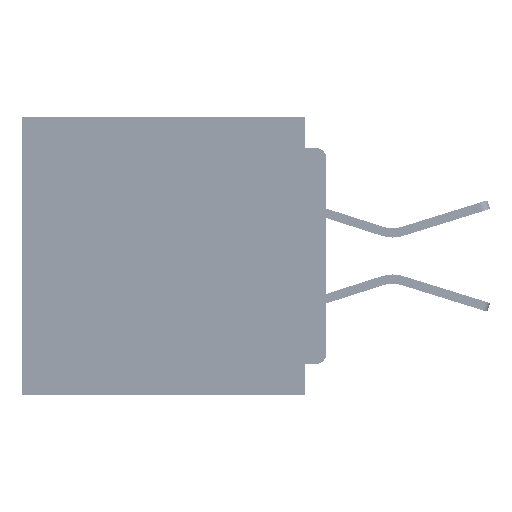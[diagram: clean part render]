
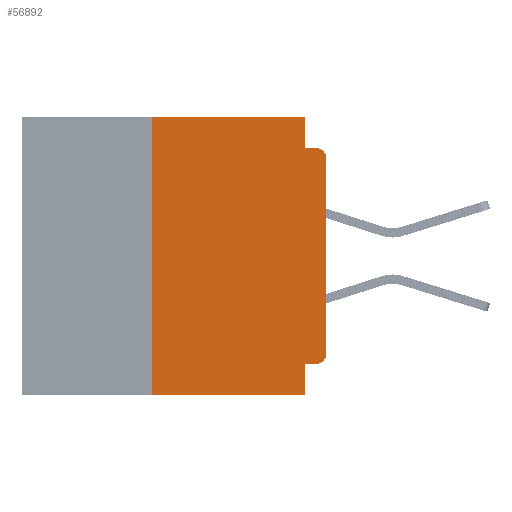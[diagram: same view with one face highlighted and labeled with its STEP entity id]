
A CAD part, left-side view. The second image highlights one B-rep face of the part: STEP entity #56892.
In plain terms, the highlighted planar face has unit normal (-1, 0, 0).
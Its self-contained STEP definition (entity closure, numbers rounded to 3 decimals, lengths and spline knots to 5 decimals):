
#153 = EDGE_CURVE ( 'NONE', #24919, #8494, #25600, .T. ) ;
#1787 = LINE ( 'NONE', #19563, #43890 ) ;
#3131 = DIRECTION ( 'NONE',  ( 0., -1., 0. ) ) ;
#3203 = CARTESIAN_POINT ( 'NONE',  ( 0., 0.437, 0. ) ) ;
#5360 = CARTESIAN_POINT ( 'NONE',  ( 0., 0., -0.06 ) ) ;
#7212 = DIRECTION ( 'NONE',  ( -1., 0., 0. ) ) ;
#7640 = EDGE_CURVE ( 'NONE', #46622, #62205, #57290, .T. ) ;
#7871 = CARTESIAN_POINT ( 'NONE',  ( 0., 0., 0. ) ) ;
#8494 = VERTEX_POINT ( 'NONE', #47604 ) ;
#9558 = LINE ( 'NONE', #55888, #34312 ) ;
#9889 = VECTOR ( 'NONE', #3131, 39.37008 ) ;
#11224 = ORIENTED_EDGE ( 'NONE', *, *, #20095, .T. ) ;
#13734 = CARTESIAN_POINT ( 'NONE',  ( 0., 0.031, -0.355 ) ) ;
#14409 = DIRECTION ( 'NONE',  ( -1., 0., 0. ) ) ;
#14825 = VERTEX_POINT ( 'NONE', #50760 ) ;
#15659 = DIRECTION ( 'NONE',  ( 0., 0., 1. ) ) ;
#16068 = ORIENTED_EDGE ( 'NONE', *, *, #51046, .F. ) ;
#18421 = AXIS2_PLACEMENT_3D ( 'NONE', #45897, #14409, #51181 ) ;
#18932 = EDGE_CURVE ( 'NONE', #21738, #14825, #9558, .T. ) ;
#19563 = CARTESIAN_POINT ( 'NONE',  ( 0., 0.031, 0. ) ) ;
#20095 = EDGE_CURVE ( 'NONE', #62205, #37852, #68107, .T. ) ;
#21738 = VERTEX_POINT ( 'NONE', #13734 ) ;
#22827 = VERTEX_POINT ( 'NONE', #33653 ) ;
#24545 = EDGE_LOOP ( 'NONE', ( #31133, #11224, #66896, #27569, #51561, #49930, #38140, #43102, #16068, #51711 ) ) ;
#24919 = VERTEX_POINT ( 'NONE', #26521 ) ;
#25376 = CARTESIAN_POINT ( 'NONE',  ( 0., 0.25, -0.4 ) ) ;
#25600 = LINE ( 'NONE', #3203, #9889 ) ;
#25955 = CARTESIAN_POINT ( 'NONE',  ( 0., 0.437, 0. ) ) ;
#26521 = CARTESIAN_POINT ( 'NONE',  ( 0., 0.25, 0. ) ) ;
#26648 = VERTEX_POINT ( 'NONE', #25376 ) ;
#26746 = EDGE_CURVE ( 'NONE', #26648, #24919, #28576, .T. ) ;
#27569 = ORIENTED_EDGE ( 'NONE', *, *, #29128, .F. ) ;
#28576 = LINE ( 'NONE', #52434, #54801 ) ;
#28652 = CARTESIAN_POINT ( 'NONE',  ( 0., 0., -0.34 ) ) ;
#29128 = EDGE_CURVE ( 'NONE', #8494, #55952, #1787, .T. ) ;
#29392 = FACE_OUTER_BOUND ( 'NONE', #24545, .T. ) ;
#29674 = VECTOR ( 'NONE', #39343, 39.37008 ) ;
#31133 = ORIENTED_EDGE ( 'NONE', *, *, #7640, .T. ) ;
#31285 = DIRECTION ( 'NONE',  ( 1., 0., 0. ) ) ;
#33653 = CARTESIAN_POINT ( 'NONE',  ( 0., 0.015, -0.355 ) ) ;
#34312 = VECTOR ( 'NONE', #35066, 39.37008 ) ;
#35066 = DIRECTION ( 'NONE',  ( 0., 0., -1. ) ) ;
#37852 = VERTEX_POINT ( 'NONE', #47292 ) ;
#38140 = ORIENTED_EDGE ( 'NONE', *, *, #43357, .T. ) ;
#38613 = DIRECTION ( 'NONE',  ( 0., -1., 0. ) ) ;
#38813 = CARTESIAN_POINT ( 'NONE',  ( 0., 0.015, -0.06 ) ) ;
#38926 = EDGE_CURVE ( 'NONE', #55952, #37852, #67020, .T. ) ;
#39343 = DIRECTION ( 'NONE',  ( 0., -1., 0. ) ) ;
#39389 = CARTESIAN_POINT ( 'NONE',  ( 0., 0.031, -0.045 ) ) ;
#39673 = DIRECTION ( 'NONE',  ( 0., 0., 1. ) ) ;
#42671 = AXIS2_PLACEMENT_3D ( 'NONE', #38813, #7212, #44038 ) ;
#43102 = ORIENTED_EDGE ( 'NONE', *, *, #18932, .F. ) ;
#43339 = VECTOR ( 'NONE', #39673, 39.37008 ) ;
#43357 = EDGE_CURVE ( 'NONE', #26648, #14825, #43586, .T. ) ;
#43586 = LINE ( 'NONE', #49887, #29674 ) ;
#43890 = VECTOR ( 'NONE', #61469, 39.37008 ) ;
#44038 = DIRECTION ( 'NONE',  ( 0., 0., -1. ) ) ;
#45897 = CARTESIAN_POINT ( 'NONE',  ( 0., 0.015, -0.34 ) ) ;
#46622 = VERTEX_POINT ( 'NONE', #28652 ) ;
#47292 = CARTESIAN_POINT ( 'NONE',  ( 0., 0.015, -0.045 ) ) ;
#47604 = CARTESIAN_POINT ( 'NONE',  ( 0., 0.031, 0. ) ) ;
#49360 = CIRCLE ( 'NONE', #18421, 0.015 ) ;
#49887 = CARTESIAN_POINT ( 'NONE',  ( 0., 0.437, -0.4 ) ) ;
#49930 = ORIENTED_EDGE ( 'NONE', *, *, #26746, .F. ) ;
#50760 = CARTESIAN_POINT ( 'NONE',  ( 0., 0.031, -0.4 ) ) ;
#51046 = EDGE_CURVE ( 'NONE', #22827, #21738, #61149, .T. ) ;
#51181 = DIRECTION ( 'NONE',  ( 0., 0., -1. ) ) ;
#51561 = ORIENTED_EDGE ( 'NONE', *, *, #153, .F. ) ;
#51711 = ORIENTED_EDGE ( 'NONE', *, *, #63897, .T. ) ;
#52434 = CARTESIAN_POINT ( 'NONE',  ( 0., 0.25, -0.4 ) ) ;
#54801 = VECTOR ( 'NONE', #15659, 39.37008 ) ;
#54809 = VECTOR ( 'NONE', #38613, 39.37008 ) ;
#55175 = CARTESIAN_POINT ( 'NONE',  ( 0., 0., -0.355 ) ) ;
#55888 = CARTESIAN_POINT ( 'NONE',  ( 0., 0.031, -0.4 ) ) ;
#55952 = VERTEX_POINT ( 'NONE', #39389 ) ;
#56813 = AXIS2_PLACEMENT_3D ( 'NONE', #25955, #31285, #67812 ) ;
#56892 = ADVANCED_FACE ( 'NONE', ( #29392 ), #57361, .F. ) ;
#57290 = LINE ( 'NONE', #7871, #43339 ) ;
#57361 = PLANE ( 'NONE',  #56813 ) ;
#59427 = CARTESIAN_POINT ( 'NONE',  ( 0., 0., -0.045 ) ) ;
#59525 = VECTOR ( 'NONE', #60660, 39.37008 ) ;
#60660 = DIRECTION ( 'NONE',  ( 0., 1., 0. ) ) ;
#61149 = LINE ( 'NONE', #55175, #59525 ) ;
#61469 = DIRECTION ( 'NONE',  ( 0., 0., -1. ) ) ;
#62205 = VERTEX_POINT ( 'NONE', #5360 ) ;
#63897 = EDGE_CURVE ( 'NONE', #22827, #46622, #49360, .T. ) ;
#66896 = ORIENTED_EDGE ( 'NONE', *, *, #38926, .F. ) ;
#67020 = LINE ( 'NONE', #59427, #54809 ) ;
#67812 = DIRECTION ( 'NONE',  ( 0., 0., -1. ) ) ;
#68107 = CIRCLE ( 'NONE', #42671, 0.015 ) ;
